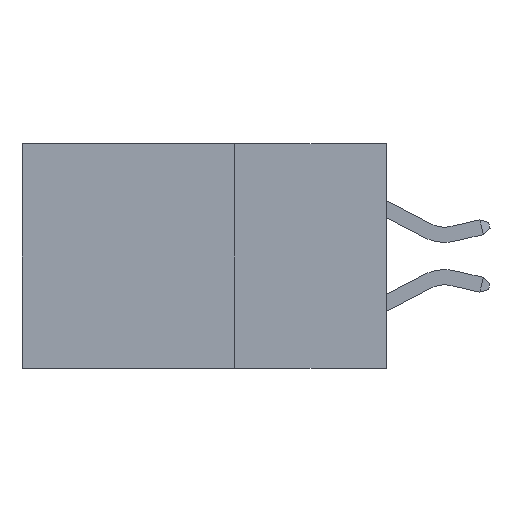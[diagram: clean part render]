
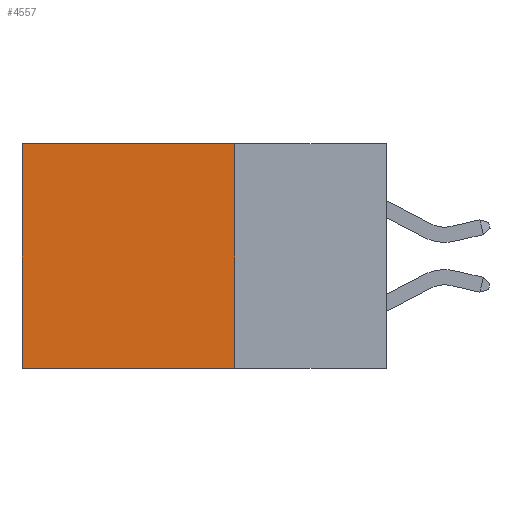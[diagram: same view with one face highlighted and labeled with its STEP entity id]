
A CAD part, left-side view. The second image highlights one B-rep face of the part: STEP entity #4557.
In plain terms, the highlighted planar face has unit normal (-1, 0, 0).
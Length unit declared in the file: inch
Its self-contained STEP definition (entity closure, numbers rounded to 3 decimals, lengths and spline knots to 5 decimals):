
#230 = AXIS2_PLACEMENT_3D ( 'NONE', #11901, #1542, #8771 ) ;
#273 = EDGE_CURVE ( 'NONE', #2492, #4827, #6133, .T. ) ;
#1161 = LINE ( 'NONE', #7643, #3678 ) ;
#1542 = DIRECTION ( 'NONE',  ( 1., 0., 0. ) ) ;
#1718 = CARTESIAN_POINT ( 'NONE',  ( 0.2615, 0.25, 0. ) ) ;
#2039 = DIRECTION ( 'NONE',  ( 0., 0., -1. ) ) ;
#2492 = VERTEX_POINT ( 'NONE', #9347 ) ;
#2499 = VERTEX_POINT ( 'NONE', #7309 ) ;
#2522 = EDGE_LOOP ( 'NONE', ( #2556, #3602, #2784, #12835 ) ) ;
#2556 = ORIENTED_EDGE ( 'NONE', *, *, #6955, .T. ) ;
#2659 = EDGE_CURVE ( 'NONE', #4827, #9366, #1161, .T. ) ;
#2784 = ORIENTED_EDGE ( 'NONE', *, *, #273, .F. ) ;
#3074 = CARTESIAN_POINT ( 'NONE',  ( 0.2615, 0.6, -0.37 ) ) ;
#3602 = ORIENTED_EDGE ( 'NONE', *, *, #2659, .F. ) ;
#3678 = VECTOR ( 'NONE', #11794, 39.37008 ) ;
#4557 = ADVANCED_FACE ( 'NONE', ( #8844 ), #5731, .F. ) ;
#4827 = VERTEX_POINT ( 'NONE', #9301 ) ;
#5586 = DIRECTION ( 'NONE',  ( 0., 0., -1. ) ) ;
#5731 = PLANE ( 'NONE',  #230 ) ;
#6133 = LINE ( 'NONE', #9243, #8388 ) ;
#6851 = LINE ( 'NONE', #1718, #10250 ) ;
#6955 = EDGE_CURVE ( 'NONE', #2499, #9366, #12336, .T. ) ;
#7309 = CARTESIAN_POINT ( 'NONE',  ( 0.2615, 0.6, 0. ) ) ;
#7643 = CARTESIAN_POINT ( 'NONE',  ( 0.2615, 0.25, -0.37 ) ) ;
#8388 = VECTOR ( 'NONE', #5586, 39.37008 ) ;
#8771 = DIRECTION ( 'NONE',  ( 0., 0., -1. ) ) ;
#8844 = FACE_OUTER_BOUND ( 'NONE', #2522, .T. ) ;
#9243 = CARTESIAN_POINT ( 'NONE',  ( 0.2615, 0.25, -0.37 ) ) ;
#9301 = CARTESIAN_POINT ( 'NONE',  ( 0.2615, 0.25, -0.37 ) ) ;
#9347 = CARTESIAN_POINT ( 'NONE',  ( 0.2615, 0.25, 0. ) ) ;
#9366 = VERTEX_POINT ( 'NONE', #12255 ) ;
#10125 = EDGE_CURVE ( 'NONE', #2492, #2499, #6851, .T. ) ;
#10237 = DIRECTION ( 'NONE',  ( 0., 1., 0. ) ) ;
#10250 = VECTOR ( 'NONE', #10237, 39.37008 ) ;
#11794 = DIRECTION ( 'NONE',  ( 0., 1., 0. ) ) ;
#11901 = CARTESIAN_POINT ( 'NONE',  ( 0.2615, 0.25, -0.37 ) ) ;
#12255 = CARTESIAN_POINT ( 'NONE',  ( 0.2615, 0.6, -0.37 ) ) ;
#12336 = LINE ( 'NONE', #3074, #13242 ) ;
#12835 = ORIENTED_EDGE ( 'NONE', *, *, #10125, .T. ) ;
#13242 = VECTOR ( 'NONE', #2039, 39.37008 ) ;
